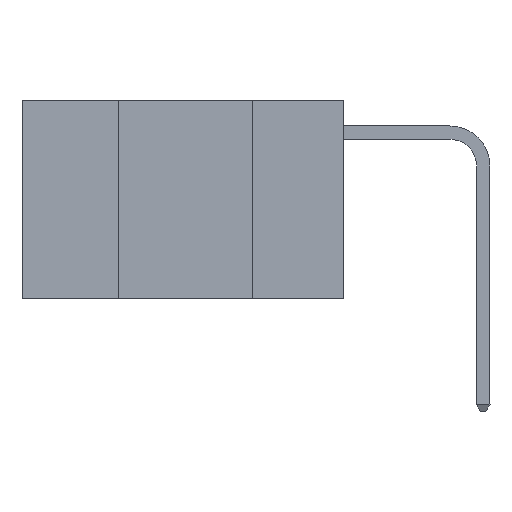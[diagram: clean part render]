
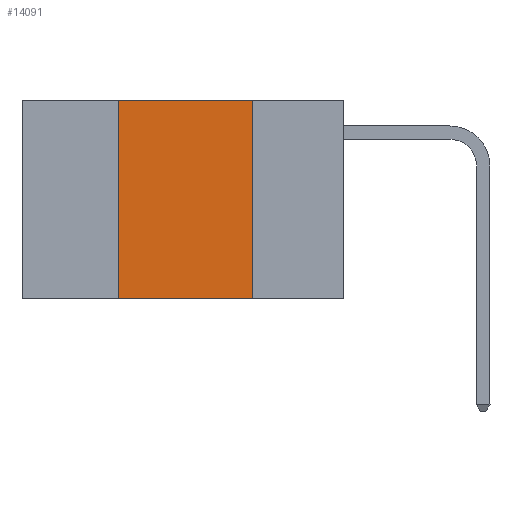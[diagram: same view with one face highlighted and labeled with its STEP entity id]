
A CAD part, left-side view. The second image highlights one B-rep face of the part: STEP entity #14091.
In plain terms, the highlighted planar face has unit normal (-1, 0, 0).
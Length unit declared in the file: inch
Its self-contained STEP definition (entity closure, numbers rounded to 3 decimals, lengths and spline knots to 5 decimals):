
#83 = ORIENTED_EDGE ( 'NONE', *, *, #7037, .F. ) ;
#84 = DIRECTION ( 'NONE',  ( 0., 0., -1. ) ) ;
#400 = CARTESIAN_POINT ( 'NONE',  ( 0., 0.17, 0. ) ) ;
#805 = EDGE_LOOP ( 'NONE', ( #83, #17147, #16054, #4218 ) ) ;
#1626 = VECTOR ( 'NONE', #13069, 39.37008 ) ;
#2418 = VERTEX_POINT ( 'NONE', #5397 ) ;
#3452 = LINE ( 'NONE', #18434, #11781 ) ;
#4218 = ORIENTED_EDGE ( 'NONE', *, *, #6913, .T. ) ;
#4351 = DIRECTION ( 'NONE',  ( 0., 0., -1. ) ) ;
#4698 = CARTESIAN_POINT ( 'NONE',  ( 0., 0.42, 0. ) ) ;
#5397 = CARTESIAN_POINT ( 'NONE',  ( 0., 0.42, -0.37 ) ) ;
#6011 = FACE_OUTER_BOUND ( 'NONE', #805, .T. ) ;
#6913 = EDGE_CURVE ( 'NONE', #2418, #14850, #19357, .T. ) ;
#7037 = EDGE_CURVE ( 'NONE', #16647, #14850, #3452, .T. ) ;
#7534 = LINE ( 'NONE', #9139, #20316 ) ;
#8031 = CARTESIAN_POINT ( 'NONE',  ( 0., 0.17, -0.37 ) ) ;
#8853 = EDGE_CURVE ( 'NONE', #2418, #12425, #10651, .T. ) ;
#9139 = CARTESIAN_POINT ( 'NONE',  ( 0., 0.6, 0. ) ) ;
#10651 = LINE ( 'NONE', #4698, #19008 ) ;
#10832 = DIRECTION ( 'NONE',  ( 0., -1., 0. ) ) ;
#11409 = DIRECTION ( 'NONE',  ( 0., 0., 1. ) ) ;
#11781 = VECTOR ( 'NONE', #84, 39.37008 ) ;
#12425 = VERTEX_POINT ( 'NONE', #13495 ) ;
#12653 = PLANE ( 'NONE',  #19854 ) ;
#13069 = DIRECTION ( 'NONE',  ( 0., -1., 0. ) ) ;
#13495 = CARTESIAN_POINT ( 'NONE',  ( 0., 0.42, 0. ) ) ;
#14091 = ADVANCED_FACE ( 'NONE', ( #6011 ), #12653, .F. ) ;
#14328 = DIRECTION ( 'NONE',  ( 1., 0., 0. ) ) ;
#14850 = VERTEX_POINT ( 'NONE', #8031 ) ;
#16054 = ORIENTED_EDGE ( 'NONE', *, *, #8853, .F. ) ;
#16455 = CARTESIAN_POINT ( 'NONE',  ( 0., 0.6, -0.37 ) ) ;
#16647 = VERTEX_POINT ( 'NONE', #400 ) ;
#17147 = ORIENTED_EDGE ( 'NONE', *, *, #21627, .F. ) ;
#18434 = CARTESIAN_POINT ( 'NONE',  ( 0., 0.17, 0. ) ) ;
#19008 = VECTOR ( 'NONE', #11409, 39.37008 ) ;
#19308 = CARTESIAN_POINT ( 'NONE',  ( 0., 0.6, 0. ) ) ;
#19357 = LINE ( 'NONE', #16455, #1626 ) ;
#19854 = AXIS2_PLACEMENT_3D ( 'NONE', #19308, #14328, #4351 ) ;
#20316 = VECTOR ( 'NONE', #10832, 39.37008 ) ;
#21627 = EDGE_CURVE ( 'NONE', #12425, #16647, #7534, .T. ) ;
